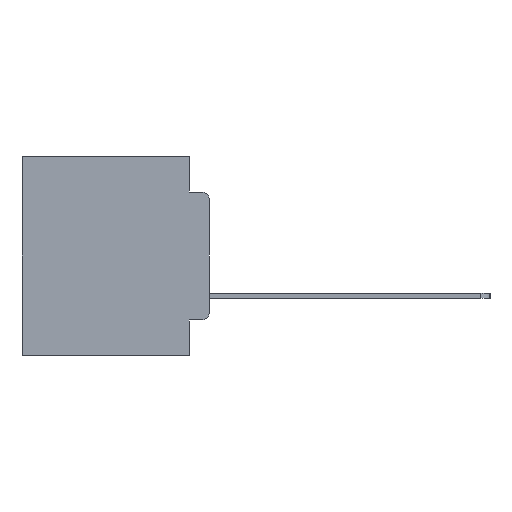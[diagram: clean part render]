
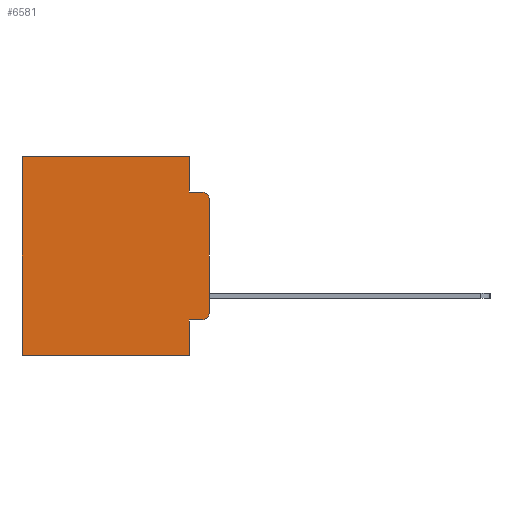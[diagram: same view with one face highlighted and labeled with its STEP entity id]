
A CAD part, left-side view. The second image highlights one B-rep face of the part: STEP entity #6581.
In plain terms, the highlighted planar face has unit normal (-1, 0, 0).
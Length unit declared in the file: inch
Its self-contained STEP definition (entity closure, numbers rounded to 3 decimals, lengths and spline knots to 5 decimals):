
#6 = DIRECTION ( 'NONE',  ( 0., 0., -1. ) ) ;
#244 = CARTESIAN_POINT ( 'NONE',  ( 0.298, 0.051, -0.5 ) ) ;
#1023 = VECTOR ( 'NONE', #2665, 39.37008 ) ;
#1735 = VERTEX_POINT ( 'NONE', #244 ) ;
#2205 = FACE_OUTER_BOUND ( 'NONE', #20793, .T. ) ;
#2230 = LINE ( 'NONE', #19290, #7162 ) ;
#2281 = LINE ( 'NONE', #16142, #7204 ) ;
#2425 = CARTESIAN_POINT ( 'NONE',  ( 0.298, 0.02, -0.1085 ) ) ;
#2468 = VECTOR ( 'NONE', #20335, 39.37008 ) ;
#2652 = VECTOR ( 'NONE', #15910, 39.37008 ) ;
#2665 = DIRECTION ( 'NONE',  ( 0., 1., 0. ) ) ;
#3051 = VERTEX_POINT ( 'NONE', #24580 ) ;
#3133 = LINE ( 'NONE', #10984, #2468 ) ;
#3220 = VERTEX_POINT ( 'NONE', #19588 ) ;
#3483 = AXIS2_PLACEMENT_3D ( 'NONE', #13404, #9598, #22701 ) ;
#3548 = VERTEX_POINT ( 'NONE', #15051 ) ;
#3814 = ORIENTED_EDGE ( 'NONE', *, *, #15904, .F. ) ;
#4071 = LINE ( 'NONE', #22132, #19027 ) ;
#4134 = CARTESIAN_POINT ( 'NONE',  ( 0.298, 0., -0.3915 ) ) ;
#4194 = CARTESIAN_POINT ( 'NONE',  ( 0.298, 0.473, -0.5 ) ) ;
#4366 = CARTESIAN_POINT ( 'NONE',  ( 0.298, 0.051, -0.0885 ) ) ;
#4571 = DIRECTION ( 'NONE',  ( 0., 0., -1. ) ) ;
#4953 = DIRECTION ( 'NONE',  ( -1., 0., 0. ) ) ;
#5294 = VERTEX_POINT ( 'NONE', #13551 ) ;
#5782 = DIRECTION ( 'NONE',  ( 0., 0., -1. ) ) ;
#6229 = EDGE_CURVE ( 'NONE', #20038, #3051, #2230, .T. ) ;
#6474 = ORIENTED_EDGE ( 'NONE', *, *, #11408, .F. ) ;
#6581 = ADVANCED_FACE ( 'NONE', ( #2205 ), #20868, .F. ) ;
#7162 = VECTOR ( 'NONE', #5782, 39.37008 ) ;
#7204 = VECTOR ( 'NONE', #6, 39.37008 ) ;
#7590 = EDGE_CURVE ( 'NONE', #3548, #9206, #19385, .T. ) ;
#7635 = EDGE_CURVE ( 'NONE', #20038, #3548, #3133, .T. ) ;
#8115 = EDGE_CURVE ( 'NONE', #10153, #5294, #11397, .T. ) ;
#8693 = AXIS2_PLACEMENT_3D ( 'NONE', #16739, #4953, #18579 ) ;
#8909 = CARTESIAN_POINT ( 'NONE',  ( 0.298, 0.051, -0.4115 ) ) ;
#9206 = VERTEX_POINT ( 'NONE', #4194 ) ;
#9331 = ORIENTED_EDGE ( 'NONE', *, *, #6229, .F. ) ;
#9598 = DIRECTION ( 'NONE',  ( 1., 0., 0. ) ) ;
#10153 = VERTEX_POINT ( 'NONE', #20345 ) ;
#10546 = ORIENTED_EDGE ( 'NONE', *, *, #7590, .T. ) ;
#10823 = DIRECTION ( 'NONE',  ( 0., 0., -1. ) ) ;
#10855 = VECTOR ( 'NONE', #16219, 39.37008 ) ;
#10984 = CARTESIAN_POINT ( 'NONE',  ( 0.298, 0., 0. ) ) ;
#11397 = CIRCLE ( 'NONE', #20955, 0.02 ) ;
#11408 = EDGE_CURVE ( 'NONE', #18863, #1735, #4071, .T. ) ;
#11686 = EDGE_CURVE ( 'NONE', #1735, #9206, #21878, .T. ) ;
#12714 = EDGE_CURVE ( 'NONE', #18863, #3220, #18961, .T. ) ;
#13404 = CARTESIAN_POINT ( 'NONE',  ( 0.298, 0., 0. ) ) ;
#13551 = CARTESIAN_POINT ( 'NONE',  ( 0.298, 0.02, -0.0885 ) ) ;
#14041 = EDGE_CURVE ( 'NONE', #3220, #21168, #23193, .T. ) ;
#14472 = VECTOR ( 'NONE', #10823, 39.37008 ) ;
#15051 = CARTESIAN_POINT ( 'NONE',  ( 0.298, 0.473, 0. ) ) ;
#15067 = ORIENTED_EDGE ( 'NONE', *, *, #7635, .T. ) ;
#15368 = LINE ( 'NONE', #4366, #10855 ) ;
#15904 = EDGE_CURVE ( 'NONE', #3051, #5294, #15368, .T. ) ;
#15910 = DIRECTION ( 'NONE',  ( 0., -1., 0. ) ) ;
#16142 = CARTESIAN_POINT ( 'NONE',  ( 0.298, 0., 0. ) ) ;
#16219 = DIRECTION ( 'NONE',  ( 0., -1., 0. ) ) ;
#16406 = DIRECTION ( 'NONE',  ( -1., 0., 0. ) ) ;
#16739 = CARTESIAN_POINT ( 'NONE',  ( 0.298, 0.02, -0.3915 ) ) ;
#16824 = ORIENTED_EDGE ( 'NONE', *, *, #12714, .T. ) ;
#17407 = ORIENTED_EDGE ( 'NONE', *, *, #14041, .T. ) ;
#17695 = ORIENTED_EDGE ( 'NONE', *, *, #8115, .T. ) ;
#17785 = CARTESIAN_POINT ( 'NONE',  ( 0.298, 0.051, -0.4115 ) ) ;
#18452 = CARTESIAN_POINT ( 'NONE',  ( 0.298, 0., -0.5 ) ) ;
#18579 = DIRECTION ( 'NONE',  ( 0., 0., -1. ) ) ;
#18863 = VERTEX_POINT ( 'NONE', #8909 ) ;
#18961 = LINE ( 'NONE', #17785, #2652 ) ;
#19027 = VECTOR ( 'NONE', #23927, 39.37008 ) ;
#19290 = CARTESIAN_POINT ( 'NONE',  ( 0.298, 0.051, 0. ) ) ;
#19385 = LINE ( 'NONE', #23816, #14472 ) ;
#19588 = CARTESIAN_POINT ( 'NONE',  ( 0.298, 0.02, -0.4115 ) ) ;
#20038 = VERTEX_POINT ( 'NONE', #21315 ) ;
#20335 = DIRECTION ( 'NONE',  ( 0., 1., 0. ) ) ;
#20345 = CARTESIAN_POINT ( 'NONE',  ( 0.298, 0., -0.1085 ) ) ;
#20538 = ORIENTED_EDGE ( 'NONE', *, *, #11686, .F. ) ;
#20793 = EDGE_LOOP ( 'NONE', ( #21952, #17695, #3814, #9331, #15067, #10546, #20538, #6474, #16824, #17407 ) ) ;
#20868 = PLANE ( 'NONE',  #3483 ) ;
#20955 = AXIS2_PLACEMENT_3D ( 'NONE', #2425, #16406, #4571 ) ;
#21168 = VERTEX_POINT ( 'NONE', #4134 ) ;
#21315 = CARTESIAN_POINT ( 'NONE',  ( 0.298, 0.051, 0. ) ) ;
#21878 = LINE ( 'NONE', #18452, #1023 ) ;
#21952 = ORIENTED_EDGE ( 'NONE', *, *, #24868, .F. ) ;
#22132 = CARTESIAN_POINT ( 'NONE',  ( 0.298, 0.051, 0. ) ) ;
#22701 = DIRECTION ( 'NONE',  ( 0., 0., -1. ) ) ;
#23193 = CIRCLE ( 'NONE', #8693, 0.02 ) ;
#23816 = CARTESIAN_POINT ( 'NONE',  ( 0.298, 0.473, 0. ) ) ;
#23927 = DIRECTION ( 'NONE',  ( 0., 0., -1. ) ) ;
#24580 = CARTESIAN_POINT ( 'NONE',  ( 0.298, 0.051, -0.0885 ) ) ;
#24868 = EDGE_CURVE ( 'NONE', #10153, #21168, #2281, .T. ) ;
